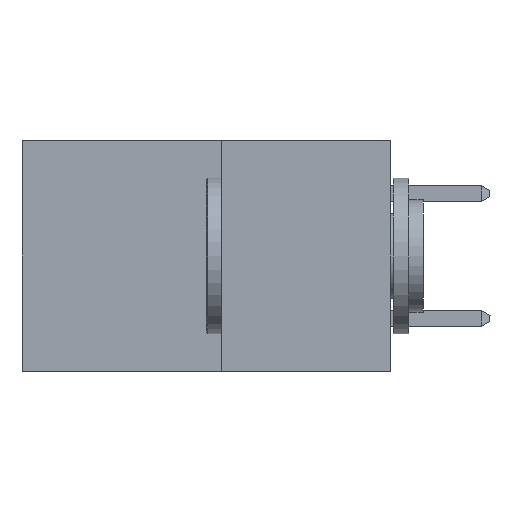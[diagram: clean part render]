
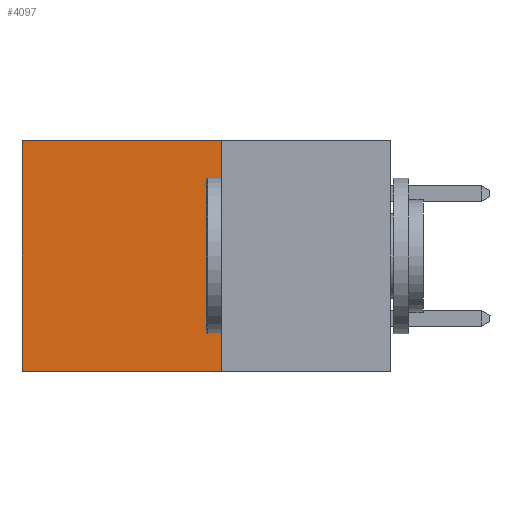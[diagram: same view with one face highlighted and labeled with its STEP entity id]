
A CAD part, left-side view. The second image highlights one B-rep face of the part: STEP entity #4097.
In plain terms, the highlighted planar face has unit normal (-1, 0, 0).
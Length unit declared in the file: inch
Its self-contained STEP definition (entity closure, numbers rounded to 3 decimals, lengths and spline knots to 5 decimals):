
#297 = FACE_OUTER_BOUND ( 'NONE', #1849, .T. ) ;
#660 = DIRECTION ( 'NONE',  ( 0., 0., -1. ) ) ;
#819 = EDGE_CURVE ( 'NONE', #8652, #3720, #1177, .T. ) ;
#1118 = DIRECTION ( 'NONE',  ( 0., 1., 0. ) ) ;
#1177 = LINE ( 'NONE', #6029, #8100 ) ;
#1849 = EDGE_LOOP ( 'NONE', ( #3941, #4495, #4808, #5509 ) ) ;
#1939 = VECTOR ( 'NONE', #6398, 39.37008 ) ;
#2015 = CARTESIAN_POINT ( 'NONE',  ( 0.277, 0.27, 0. ) ) ;
#2600 = EDGE_CURVE ( 'NONE', #3720, #4064, #7073, .T. ) ;
#3038 = CARTESIAN_POINT ( 'NONE',  ( 0.277, 0.59, -0.37 ) ) ;
#3054 = PLANE ( 'NONE',  #11433 ) ;
#3181 = DIRECTION ( 'NONE',  ( 1., 0., 0. ) ) ;
#3720 = VERTEX_POINT ( 'NONE', #5095 ) ;
#3941 = ORIENTED_EDGE ( 'NONE', *, *, #2600, .T. ) ;
#4064 = VERTEX_POINT ( 'NONE', #3038 ) ;
#4078 = VERTEX_POINT ( 'NONE', #5451 ) ;
#4097 = ADVANCED_FACE ( 'NONE', ( #297 ), #3054, .F. ) ;
#4274 = CARTESIAN_POINT ( 'NONE',  ( 0.277, 0.27, -0.37 ) ) ;
#4406 = DIRECTION ( 'NONE',  ( 0., 0., -1. ) ) ;
#4495 = ORIENTED_EDGE ( 'NONE', *, *, #5885, .F. ) ;
#4808 = ORIENTED_EDGE ( 'NONE', *, *, #11582, .F. ) ;
#5095 = CARTESIAN_POINT ( 'NONE',  ( 0.277, 0.59, 0. ) ) ;
#5451 = CARTESIAN_POINT ( 'NONE',  ( 0.277, 0.27, -0.37 ) ) ;
#5461 = LINE ( 'NONE', #8939, #7600 ) ;
#5509 = ORIENTED_EDGE ( 'NONE', *, *, #819, .T. ) ;
#5885 = EDGE_CURVE ( 'NONE', #4078, #4064, #11275, .T. ) ;
#5912 = CARTESIAN_POINT ( 'NONE',  ( 0.277, 0.59, -0.37 ) ) ;
#6029 = CARTESIAN_POINT ( 'NONE',  ( 0.277, 0.27, 0. ) ) ;
#6398 = DIRECTION ( 'NONE',  ( 0., 1., 0. ) ) ;
#6613 = CARTESIAN_POINT ( 'NONE',  ( 0.277, 0.27, -0.37 ) ) ;
#7073 = LINE ( 'NONE', #5912, #8918 ) ;
#7600 = VECTOR ( 'NONE', #4406, 39.37008 ) ;
#8100 = VECTOR ( 'NONE', #1118, 39.37008 ) ;
#8652 = VERTEX_POINT ( 'NONE', #2015 ) ;
#8918 = VECTOR ( 'NONE', #9510, 39.37008 ) ;
#8939 = CARTESIAN_POINT ( 'NONE',  ( 0.277, 0.27, -0.37 ) ) ;
#9510 = DIRECTION ( 'NONE',  ( 0., 0., -1. ) ) ;
#11275 = LINE ( 'NONE', #6613, #1939 ) ;
#11433 = AXIS2_PLACEMENT_3D ( 'NONE', #4274, #3181, #660 ) ;
#11582 = EDGE_CURVE ( 'NONE', #8652, #4078, #5461, .T. ) ;
